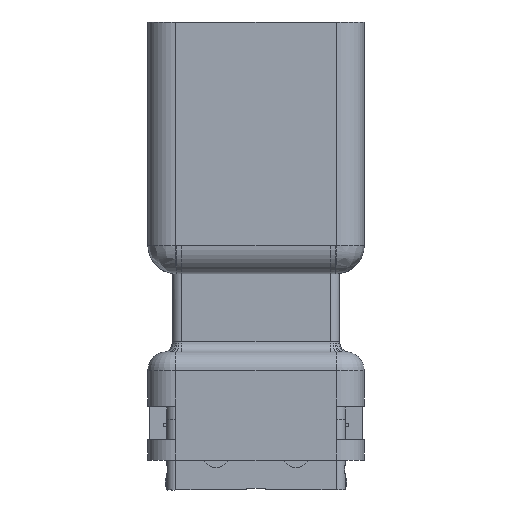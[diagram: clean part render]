
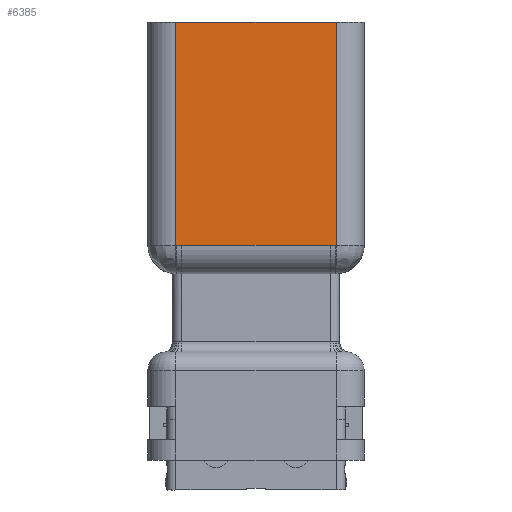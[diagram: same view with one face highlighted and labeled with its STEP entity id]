
A CAD part, front view. The second image highlights one B-rep face of the part: STEP entity #6385.
In plain terms, the highlighted planar face has unit normal (0, -1, 0).
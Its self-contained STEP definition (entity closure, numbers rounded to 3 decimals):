
#586 = DIRECTION ( 'NONE',  ( 0., 1., 0. ) ) ;
#606 = CARTESIAN_POINT ( 'NONE',  ( -4.3, -3.975, 13.5 ) ) ;
#1277 = DIRECTION ( 'NONE',  ( 0., 0., -1. ) ) ;
#1462 = VECTOR ( 'NONE', #1277, 1000. ) ;
#1517 = CARTESIAN_POINT ( 'NONE',  ( -4.156, -3.975, 1.53 ) ) ;
#2199 = CARTESIAN_POINT ( 'NONE',  ( 4.063, -3.975, 1.528 ) ) ;
#2331 = VERTEX_POINT ( 'NONE', #10321 ) ;
#2635 = CARTESIAN_POINT ( 'NONE',  ( -4.063, -3.975, 1.528 ) ) ;
#2830 = LINE ( 'NONE', #11811, #1462 ) ;
#2953 = EDGE_LOOP ( 'NONE', ( #14772, #10089, #3345, #4436, #9425, #9997, #3628, #7738 ) ) ;
#3345 = ORIENTED_EDGE ( 'NONE', *, *, #8426, .T. ) ;
#3411 = CARTESIAN_POINT ( 'NONE',  ( -4.249, -3.975, 1.53 ) ) ;
#3628 = ORIENTED_EDGE ( 'NONE', *, *, #11871, .F. ) ;
#3925 = VECTOR ( 'NONE', #6781, 1000. ) ;
#4416 = VERTEX_POINT ( 'NONE', #9073 ) ;
#4436 = ORIENTED_EDGE ( 'NONE', *, *, #9079, .T. ) ;
#4550 = CARTESIAN_POINT ( 'NONE',  ( 3.97, -3.975, 1.528 ) ) ;
#4591 = EDGE_CURVE ( 'NONE', #7425, #9013, #7235, .T. ) ;
#4869 = VECTOR ( 'NONE', #12669, 1000. ) ;
#5422 = CARTESIAN_POINT ( 'NONE',  ( 3.97, -3.975, 1.528 ) ) ;
#5689 = VECTOR ( 'NONE', #5991, 1000. ) ;
#5991 = DIRECTION ( 'NONE',  ( 1., 0., 0. ) ) ;
#6172 = CARTESIAN_POINT ( 'NONE',  ( 4.249, -3.975, 1.53 ) ) ;
#6385 = ADVANCED_FACE ( 'NONE', ( #12399 ), #13348, .F. ) ;
#6435 = CARTESIAN_POINT ( 'NONE',  ( -4.3, -3.975, 1.53 ) ) ;
#6462 = B_SPLINE_CURVE_WITH_KNOTS ( 'NONE', 3,
 ( #8098, #1517, #2635, #10772 ),
 .UNSPECIFIED., .F., .F.,
 ( 4, 4 ),
 ( 0., 0. ),
 .UNSPECIFIED. ) ;
#6781 = DIRECTION ( 'NONE',  ( 1., 0., 0. ) ) ;
#7235 = B_SPLINE_CURVE_WITH_KNOTS ( 'NONE', 3,
 ( #4550, #2199, #16621, #6172 ),
 .UNSPECIFIED., .F., .F.,
 ( 4, 4 ),
 ( 0., 0. ),
 .UNSPECIFIED. ) ;
#7425 = VERTEX_POINT ( 'NONE', #5422 ) ;
#7738 = ORIENTED_EDGE ( 'NONE', *, *, #14676, .F. ) ;
#8093 = LINE ( 'NONE', #6435, #3925 ) ;
#8098 = CARTESIAN_POINT ( 'NONE',  ( -4.249, -3.975, 1.53 ) ) ;
#8207 = DIRECTION ( 'NONE',  ( 1., 0., 0. ) ) ;
#8276 = CARTESIAN_POINT ( 'NONE',  ( -4.3, -3.975, 13.5 ) ) ;
#8426 = EDGE_CURVE ( 'NONE', #9644, #14714, #6462, .T. ) ;
#8633 = CARTESIAN_POINT ( 'NONE',  ( -4.3, -3.975, 13.5 ) ) ;
#8717 = LINE ( 'NONE', #8633, #4869 ) ;
#8757 = LINE ( 'NONE', #11349, #5689 ) ;
#9013 = VERTEX_POINT ( 'NONE', #12460 ) ;
#9073 = CARTESIAN_POINT ( 'NONE',  ( 4.3, -3.975, 13.5 ) ) ;
#9079 = EDGE_CURVE ( 'NONE', #14714, #7425, #8757, .T. ) ;
#9284 = EDGE_CURVE ( 'NONE', #2331, #12202, #8717, .T. ) ;
#9400 = VECTOR ( 'NONE', #8207, 1000. ) ;
#9425 = ORIENTED_EDGE ( 'NONE', *, *, #4591, .T. ) ;
#9644 = VERTEX_POINT ( 'NONE', #3411 ) ;
#9997 = ORIENTED_EDGE ( 'NONE', *, *, #10734, .T. ) ;
#10089 = ORIENTED_EDGE ( 'NONE', *, *, #15248, .T. ) ;
#10321 = CARTESIAN_POINT ( 'NONE',  ( -4.3, -3.975, 13.5 ) ) ;
#10734 = EDGE_CURVE ( 'NONE', #9013, #12619, #8093, .T. ) ;
#10772 = CARTESIAN_POINT ( 'NONE',  ( -3.97, -3.975, 1.528 ) ) ;
#11132 = DIRECTION ( 'NONE',  ( 0., 0., 1. ) ) ;
#11289 = CARTESIAN_POINT ( 'NONE',  ( -4.3, -3.975, 1.53 ) ) ;
#11349 = CARTESIAN_POINT ( 'NONE',  ( -4.3, -3.975, 1.528 ) ) ;
#11811 = CARTESIAN_POINT ( 'NONE',  ( 4.3, -3.975, 13.5 ) ) ;
#11871 = EDGE_CURVE ( 'NONE', #4416, #12619, #2830, .T. ) ;
#12166 = CARTESIAN_POINT ( 'NONE',  ( -3.97, -3.975, 1.528 ) ) ;
#12202 = VERTEX_POINT ( 'NONE', #16635 ) ;
#12399 = FACE_OUTER_BOUND ( 'NONE', #2953, .T. ) ;
#12415 = LINE ( 'NONE', #606, #9400 ) ;
#12460 = CARTESIAN_POINT ( 'NONE',  ( 4.249, -3.975, 1.53 ) ) ;
#12559 = CARTESIAN_POINT ( 'NONE',  ( 4.3, -3.975, 1.53 ) ) ;
#12619 = VERTEX_POINT ( 'NONE', #12559 ) ;
#12648 = DIRECTION ( 'NONE',  ( 1., 0., 0. ) ) ;
#12669 = DIRECTION ( 'NONE',  ( 0., 0., -1. ) ) ;
#13348 = PLANE ( 'NONE',  #16791 ) ;
#14676 = EDGE_CURVE ( 'NONE', #2331, #4416, #12415, .T. ) ;
#14714 = VERTEX_POINT ( 'NONE', #12166 ) ;
#14772 = ORIENTED_EDGE ( 'NONE', *, *, #9284, .T. ) ;
#15245 = LINE ( 'NONE', #11289, #16853 ) ;
#15248 = EDGE_CURVE ( 'NONE', #12202, #9644, #15245, .T. ) ;
#16621 = CARTESIAN_POINT ( 'NONE',  ( 4.156, -3.975, 1.53 ) ) ;
#16635 = CARTESIAN_POINT ( 'NONE',  ( -4.3, -3.975, 1.53 ) ) ;
#16791 = AXIS2_PLACEMENT_3D ( 'NONE', #8276, #586, #11132 ) ;
#16853 = VECTOR ( 'NONE', #12648, 1000. ) ;
